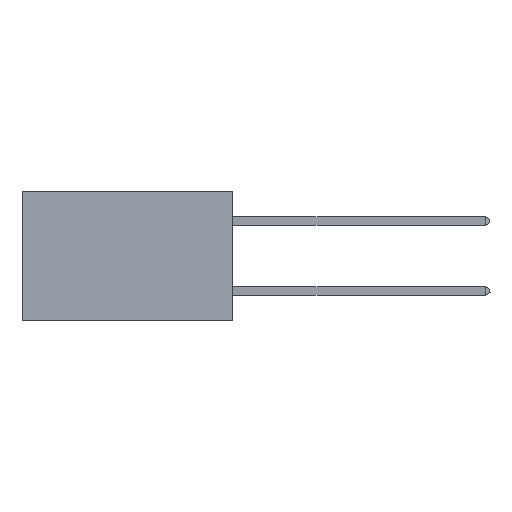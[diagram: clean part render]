
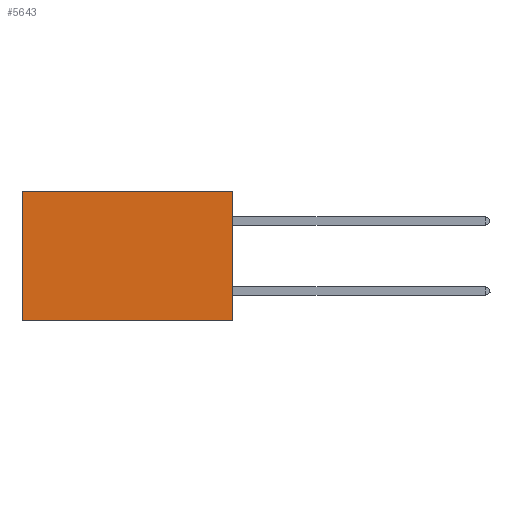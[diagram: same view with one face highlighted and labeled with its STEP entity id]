
A CAD part, left-side view. The second image highlights one B-rep face of the part: STEP entity #5643.
In plain terms, the highlighted planar face has unit normal (-1, 0, 0).
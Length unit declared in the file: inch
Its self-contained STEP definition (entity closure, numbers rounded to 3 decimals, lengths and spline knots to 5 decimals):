
#328 = ORIENTED_EDGE ( 'NONE', *, *, #2631, .T. ) ;
#567 = CARTESIAN_POINT ( 'NONE',  ( 0.2875, 0.6, -0.37 ) ) ;
#733 = CARTESIAN_POINT ( 'NONE',  ( 0.2875, 0., 0. ) ) ;
#1050 = FACE_OUTER_BOUND ( 'NONE', #8273, .T. ) ;
#1198 = VERTEX_POINT ( 'NONE', #7699 ) ;
#1846 = DIRECTION ( 'NONE',  ( 0., 0., -1. ) ) ;
#1952 = DIRECTION ( 'NONE',  ( 1., 0., 0. ) ) ;
#2445 = EDGE_CURVE ( 'NONE', #9582, #11027, #9458, .T. ) ;
#2631 = EDGE_CURVE ( 'NONE', #9921, #1198, #11618, .T. ) ;
#3124 = VECTOR ( 'NONE', #8102, 39.37008 ) ;
#3148 = AXIS2_PLACEMENT_3D ( 'NONE', #733, #1952, #1846 ) ;
#3230 = DIRECTION ( 'NONE',  ( 0., 0., -1. ) ) ;
#4896 = ORIENTED_EDGE ( 'NONE', *, *, #11953, .F. ) ;
#4964 = LINE ( 'NONE', #8918, #8148 ) ;
#4994 = VECTOR ( 'NONE', #3230, 39.37008 ) ;
#5191 = ORIENTED_EDGE ( 'NONE', *, *, #12274, .T. ) ;
#5643 = ADVANCED_FACE ( 'NONE', ( #1050 ), #6101, .F. ) ;
#5747 = DIRECTION ( 'NONE',  ( 0., 0., -1. ) ) ;
#6101 = PLANE ( 'NONE',  #3148 ) ;
#6619 = CARTESIAN_POINT ( 'NONE',  ( 0.2875, 0., -0.37 ) ) ;
#7012 = CARTESIAN_POINT ( 'NONE',  ( 0.2875, 0., 0. ) ) ;
#7699 = CARTESIAN_POINT ( 'NONE',  ( 0.2875, 0.6, 0. ) ) ;
#8102 = DIRECTION ( 'NONE',  ( 0., 1., 0. ) ) ;
#8148 = VECTOR ( 'NONE', #5747, 39.37008 ) ;
#8273 = EDGE_LOOP ( 'NONE', ( #5191, #10750, #4896, #328 ) ) ;
#8918 = CARTESIAN_POINT ( 'NONE',  ( 0.2875, 0.6, 0. ) ) ;
#9458 = LINE ( 'NONE', #10990, #12286 ) ;
#9582 = VERTEX_POINT ( 'NONE', #6619 ) ;
#9921 = VERTEX_POINT ( 'NONE', #12533 ) ;
#10675 = LINE ( 'NONE', #11652, #4994 ) ;
#10750 = ORIENTED_EDGE ( 'NONE', *, *, #2445, .F. ) ;
#10990 = CARTESIAN_POINT ( 'NONE',  ( 0.2875, 0., -0.37 ) ) ;
#11027 = VERTEX_POINT ( 'NONE', #567 ) ;
#11618 = LINE ( 'NONE', #7012, #3124 ) ;
#11652 = CARTESIAN_POINT ( 'NONE',  ( 0.2875, 0., 0. ) ) ;
#11953 = EDGE_CURVE ( 'NONE', #9921, #9582, #10675, .T. ) ;
#12274 = EDGE_CURVE ( 'NONE', #1198, #11027, #4964, .T. ) ;
#12286 = VECTOR ( 'NONE', #13145, 39.37008 ) ;
#12533 = CARTESIAN_POINT ( 'NONE',  ( 0.2875, 0., 0. ) ) ;
#13145 = DIRECTION ( 'NONE',  ( 0., 1., 0. ) ) ;
